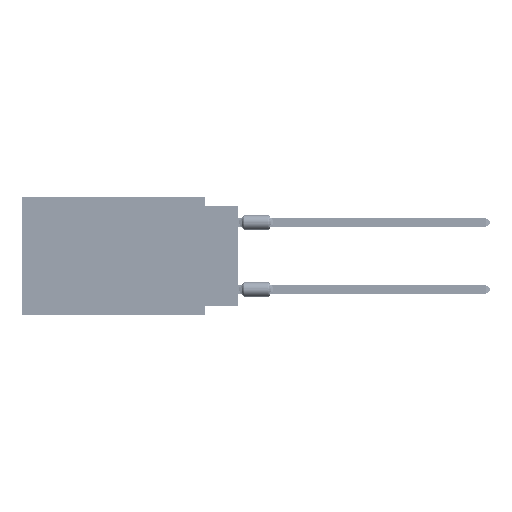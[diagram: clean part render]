
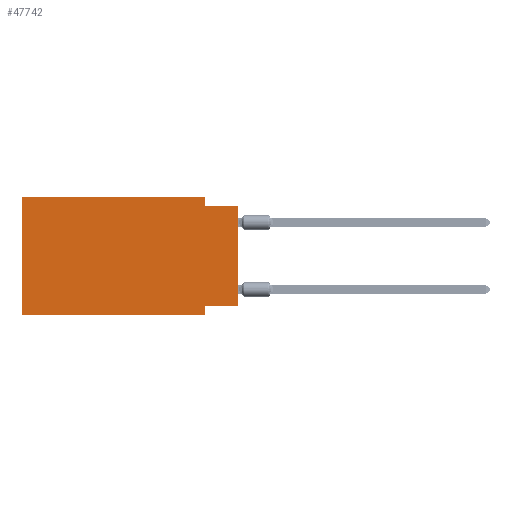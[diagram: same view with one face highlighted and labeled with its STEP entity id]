
A CAD part, left-side view. The second image highlights one B-rep face of the part: STEP entity #47742.
In plain terms, the highlighted planar face has unit normal (-1, 0, 0).
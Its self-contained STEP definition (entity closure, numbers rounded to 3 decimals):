
#479 = EDGE_CURVE ( 'NONE', #51449, #3085, #10721, .T. ) ;
#1107 = DIRECTION ( 'NONE',  ( 0., 1., 0. ) ) ;
#1325 = AXIS2_PLACEMENT_3D ( 'NONE', #79460, #72178, #13954 ) ;
#1756 = CARTESIAN_POINT ( 'NONE',  ( 0., 0., -0.635 ) ) ;
#1815 = ORIENTED_EDGE ( 'NONE', *, *, #65101, .T. ) ;
#3085 = VERTEX_POINT ( 'NONE', #62908 ) ;
#3305 = VERTEX_POINT ( 'NONE', #73958 ) ;
#5061 = EDGE_LOOP ( 'NONE', ( #1815, #30784, #46841, #35254, #26723, #23486, #32828, #17096 ) ) ;
#6167 = VECTOR ( 'NONE', #1107, 1000. ) ;
#10534 = CARTESIAN_POINT ( 'NONE',  ( 0., 2.54, 0. ) ) ;
#10721 = LINE ( 'NONE', #69360, #58865 ) ;
#12548 = EDGE_CURVE ( 'NONE', #41805, #55494, #18897, .T. ) ;
#12688 = CARTESIAN_POINT ( 'NONE',  ( 0., 0., -8.255 ) ) ;
#13954 = DIRECTION ( 'NONE',  ( 0., 0., -1. ) ) ;
#17096 = ORIENTED_EDGE ( 'NONE', *, *, #63792, .F. ) ;
#17616 = CARTESIAN_POINT ( 'NONE',  ( 0., 16.383, 0. ) ) ;
#18897 = LINE ( 'NONE', #17616, #38788 ) ;
#20492 = DIRECTION ( 'NONE',  ( 0., 0., 1. ) ) ;
#21345 = LINE ( 'NONE', #39753, #84265 ) ;
#23071 = DIRECTION ( 'NONE',  ( 0., -1., 0. ) ) ;
#23486 = ORIENTED_EDGE ( 'NONE', *, *, #39739, .T. ) ;
#24835 = CARTESIAN_POINT ( 'NONE',  ( 0., 0., -0.635 ) ) ;
#25248 = DIRECTION ( 'NONE',  ( 0., 0., -1. ) ) ;
#26723 = ORIENTED_EDGE ( 'NONE', *, *, #12548, .F. ) ;
#30784 = ORIENTED_EDGE ( 'NONE', *, *, #54332, .F. ) ;
#32828 = ORIENTED_EDGE ( 'NONE', *, *, #43481, .F. ) ;
#33219 = VECTOR ( 'NONE', #36106, 1000. ) ;
#35254 = ORIENTED_EDGE ( 'NONE', *, *, #54581, .F. ) ;
#36106 = DIRECTION ( 'NONE',  ( 0., -1., 0. ) ) ;
#38788 = VECTOR ( 'NONE', #44998, 1000. ) ;
#39739 = EDGE_CURVE ( 'NONE', #41805, #53293, #49374, .T. ) ;
#39753 = CARTESIAN_POINT ( 'NONE',  ( 0., 0., 0. ) ) ;
#40067 = LINE ( 'NONE', #12688, #6167 ) ;
#40182 = CARTESIAN_POINT ( 'NONE',  ( 0., 0., -8.255 ) ) ;
#41177 = DIRECTION ( 'NONE',  ( 0., 0., -1. ) ) ;
#41805 = VERTEX_POINT ( 'NONE', #79807 ) ;
#43481 = EDGE_CURVE ( 'NONE', #3305, #53293, #61708, .T. ) ;
#44530 = LINE ( 'NONE', #24835, #78514 ) ;
#44998 = DIRECTION ( 'NONE',  ( 0., 0., 1. ) ) ;
#45654 = FACE_OUTER_BOUND ( 'NONE', #5061, .T. ) ;
#46841 = ORIENTED_EDGE ( 'NONE', *, *, #479, .F. ) ;
#47384 = VERTEX_POINT ( 'NONE', #40182 ) ;
#47742 = ADVANCED_FACE ( 'NONE', ( #45654 ), #80308, .F. ) ;
#48660 = VERTEX_POINT ( 'NONE', #1756 ) ;
#48992 = CARTESIAN_POINT ( 'NONE',  ( 0., 16.383, 0. ) ) ;
#49374 = LINE ( 'NONE', #63486, #33219 ) ;
#51449 = VERTEX_POINT ( 'NONE', #10534 ) ;
#53293 = VERTEX_POINT ( 'NONE', #73678 ) ;
#54332 = EDGE_CURVE ( 'NONE', #3085, #48660, #44530, .T. ) ;
#54581 = EDGE_CURVE ( 'NONE', #55494, #51449, #62035, .T. ) ;
#55494 = VERTEX_POINT ( 'NONE', #48992 ) ;
#58865 = VECTOR ( 'NONE', #25248, 1000. ) ;
#61708 = LINE ( 'NONE', #72856, #76007 ) ;
#62035 = LINE ( 'NONE', #68446, #66212 ) ;
#62908 = CARTESIAN_POINT ( 'NONE',  ( 0., 2.54, -0.635 ) ) ;
#63486 = CARTESIAN_POINT ( 'NONE',  ( 0., 16.383, -8.89 ) ) ;
#63792 = EDGE_CURVE ( 'NONE', #47384, #3305, #40067, .T. ) ;
#65101 = EDGE_CURVE ( 'NONE', #47384, #48660, #21345, .T. ) ;
#66212 = VECTOR ( 'NONE', #23071, 1000. ) ;
#68446 = CARTESIAN_POINT ( 'NONE',  ( 0., 16.383, 0. ) ) ;
#69360 = CARTESIAN_POINT ( 'NONE',  ( 0., 2.54, 0. ) ) ;
#72178 = DIRECTION ( 'NONE',  ( 1., 0., 0. ) ) ;
#72856 = CARTESIAN_POINT ( 'NONE',  ( 0., 2.54, -8.89 ) ) ;
#73678 = CARTESIAN_POINT ( 'NONE',  ( 0., 2.54, -8.89 ) ) ;
#73958 = CARTESIAN_POINT ( 'NONE',  ( 0., 2.54, -8.255 ) ) ;
#76007 = VECTOR ( 'NONE', #41177, 1000. ) ;
#77082 = DIRECTION ( 'NONE',  ( 0., -1., 0. ) ) ;
#78514 = VECTOR ( 'NONE', #77082, 1000. ) ;
#79460 = CARTESIAN_POINT ( 'NONE',  ( 0., 16.383, 0. ) ) ;
#79807 = CARTESIAN_POINT ( 'NONE',  ( 0., 16.383, -8.89 ) ) ;
#80308 = PLANE ( 'NONE',  #1325 ) ;
#84265 = VECTOR ( 'NONE', #20492, 1000. ) ;
